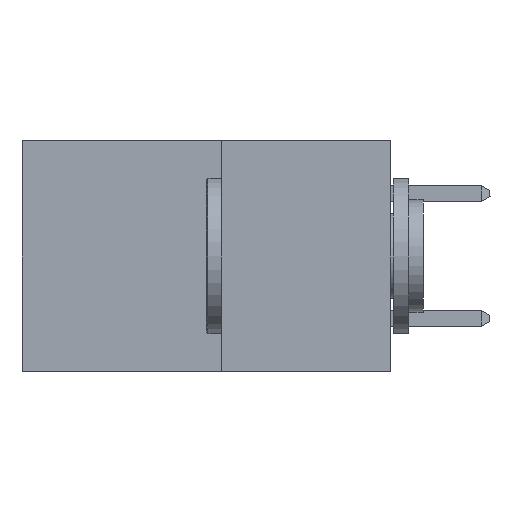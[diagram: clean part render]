
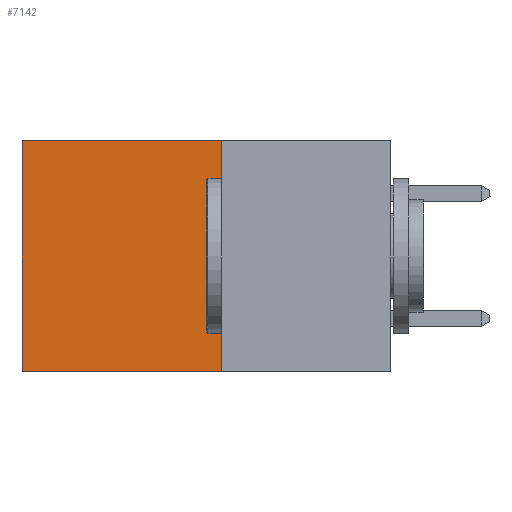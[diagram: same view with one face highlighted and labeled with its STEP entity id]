
A CAD part, left-side view. The second image highlights one B-rep face of the part: STEP entity #7142.
In plain terms, the highlighted planar face has unit normal (-1, 0, 0).
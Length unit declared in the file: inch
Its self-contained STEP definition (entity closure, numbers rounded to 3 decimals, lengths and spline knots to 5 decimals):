
#193 = CARTESIAN_POINT ( 'NONE',  ( 0.277, 0.59, -0.37 ) ) ;
#242 = EDGE_CURVE ( 'NONE', #23738, #23327, #5096, .T. ) ;
#379 = DIRECTION ( 'NONE',  ( 0., 0., -1. ) ) ;
#467 = ORIENTED_EDGE ( 'NONE', *, *, #242, .F. ) ;
#706 = CARTESIAN_POINT ( 'NONE',  ( 0.277, 0.59, -0.37 ) ) ;
#843 = LINE ( 'NONE', #23798, #25228 ) ;
#1712 = EDGE_CURVE ( 'NONE', #23738, #22253, #843, .T. ) ;
#1891 = CARTESIAN_POINT ( 'NONE',  ( 0.277, 0.27, 0. ) ) ;
#1946 = LINE ( 'NONE', #16186, #22363 ) ;
#3490 = DIRECTION ( 'NONE',  ( 0., 0., -1. ) ) ;
#4447 = VECTOR ( 'NONE', #3490, 39.37008 ) ;
#4978 = EDGE_CURVE ( 'NONE', #22253, #24678, #16649, .T. ) ;
#5096 = LINE ( 'NONE', #14992, #4447 ) ;
#5470 = DIRECTION ( 'NONE',  ( 0., 0., -1. ) ) ;
#5535 = DIRECTION ( 'NONE',  ( 1., 0., 0. ) ) ;
#5564 = PLANE ( 'NONE',  #8597 ) ;
#5605 = EDGE_CURVE ( 'NONE', #23327, #24678, #1946, .T. ) ;
#5971 = CARTESIAN_POINT ( 'NONE',  ( 0.277, 0.27, -0.37 ) ) ;
#7142 = ADVANCED_FACE ( 'NONE', ( #14724 ), #5564, .F. ) ;
#8260 = EDGE_LOOP ( 'NONE', ( #8670, #24249, #467, #16439 ) ) ;
#8597 = AXIS2_PLACEMENT_3D ( 'NONE', #5971, #5535, #5470 ) ;
#8670 = ORIENTED_EDGE ( 'NONE', *, *, #4978, .T. ) ;
#8886 = CARTESIAN_POINT ( 'NONE',  ( 0.277, 0.27, -0.37 ) ) ;
#10746 = VECTOR ( 'NONE', #379, 39.37008 ) ;
#12950 = CARTESIAN_POINT ( 'NONE',  ( 0.277, 0.59, 0. ) ) ;
#14724 = FACE_OUTER_BOUND ( 'NONE', #8260, .T. ) ;
#14992 = CARTESIAN_POINT ( 'NONE',  ( 0.277, 0.27, -0.37 ) ) ;
#15702 = DIRECTION ( 'NONE',  ( 0., 1., 0. ) ) ;
#16186 = CARTESIAN_POINT ( 'NONE',  ( 0.277, 0.27, -0.37 ) ) ;
#16439 = ORIENTED_EDGE ( 'NONE', *, *, #1712, .T. ) ;
#16649 = LINE ( 'NONE', #193, #10746 ) ;
#19283 = DIRECTION ( 'NONE',  ( 0., 1., 0. ) ) ;
#22253 = VERTEX_POINT ( 'NONE', #12950 ) ;
#22363 = VECTOR ( 'NONE', #15702, 39.37008 ) ;
#23327 = VERTEX_POINT ( 'NONE', #8886 ) ;
#23738 = VERTEX_POINT ( 'NONE', #1891 ) ;
#23798 = CARTESIAN_POINT ( 'NONE',  ( 0.277, 0.27, 0. ) ) ;
#24249 = ORIENTED_EDGE ( 'NONE', *, *, #5605, .F. ) ;
#24678 = VERTEX_POINT ( 'NONE', #706 ) ;
#25228 = VECTOR ( 'NONE', #19283, 39.37008 ) ;
